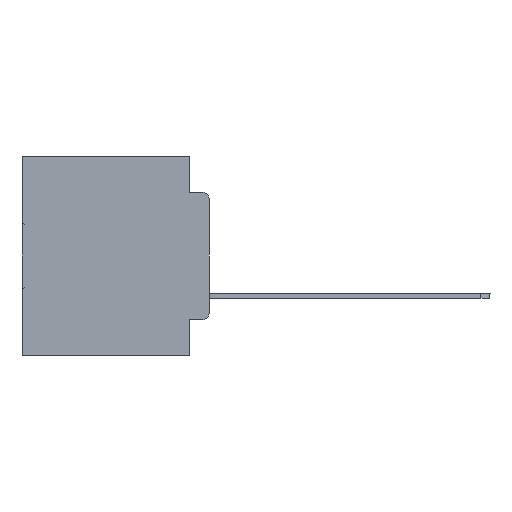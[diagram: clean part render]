
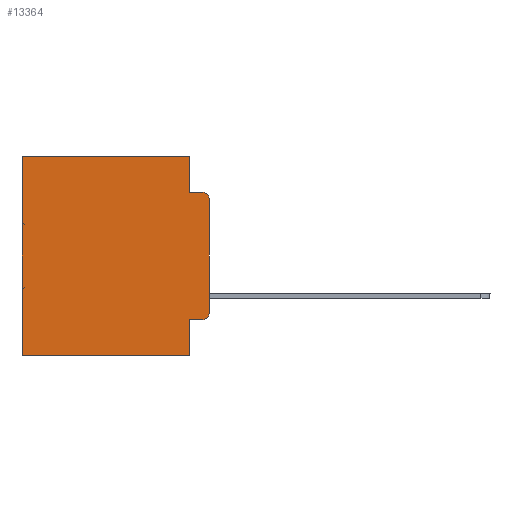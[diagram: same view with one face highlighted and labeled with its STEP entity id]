
A CAD part, left-side view. The second image highlights one B-rep face of the part: STEP entity #13364.
In plain terms, the highlighted planar face has unit normal (-1, 0, 0).
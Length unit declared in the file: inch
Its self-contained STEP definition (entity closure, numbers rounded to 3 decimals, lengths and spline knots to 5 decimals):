
#32 = LINE ( 'NONE', #24792, #26494 ) ;
#556 = ORIENTED_EDGE ( 'NONE', *, *, #33785, .F. ) ;
#729 = VECTOR ( 'NONE', #1368, 39.37008 ) ;
#1055 = DIRECTION ( 'NONE',  ( 0., 0., -1. ) ) ;
#1368 = DIRECTION ( 'NONE',  ( 0., 1., 0. ) ) ;
#2837 = LINE ( 'NONE', #18769, #14539 ) ;
#3476 = CARTESIAN_POINT ( 'NONE',  ( 0.298, 0.051, 0. ) ) ;
#3551 = CIRCLE ( 'NONE', #8074, 0.02 ) ;
#4330 = FACE_OUTER_BOUND ( 'NONE', #20759, .T. ) ;
#4646 = CARTESIAN_POINT ( 'NONE',  ( 0.298, 0.473, -0.5 ) ) ;
#4681 = AXIS2_PLACEMENT_3D ( 'NONE', #16268, #11324, #32523 ) ;
#4830 = DIRECTION ( 'NONE',  ( 1., 0., 0. ) ) ;
#4933 = CARTESIAN_POINT ( 'NONE',  ( 0.298, 0.02, -0.1085 ) ) ;
#5260 = ORIENTED_EDGE ( 'NONE', *, *, #27398, .F. ) ;
#5431 = LINE ( 'NONE', #3476, #23347 ) ;
#5491 = LINE ( 'NONE', #26901, #16795 ) ;
#6513 = VERTEX_POINT ( 'NONE', #16543 ) ;
#7020 = VERTEX_POINT ( 'NONE', #18983 ) ;
#8074 = AXIS2_PLACEMENT_3D ( 'NONE', #4933, #21043, #26337 ) ;
#9026 = CARTESIAN_POINT ( 'NONE',  ( 0.298, 0.473, 0. ) ) ;
#9737 = DIRECTION ( 'NONE',  ( 0., -1., 0. ) ) ;
#10448 = ORIENTED_EDGE ( 'NONE', *, *, #18953, .T. ) ;
#10665 = ORIENTED_EDGE ( 'NONE', *, *, #31456, .T. ) ;
#11016 = DIRECTION ( 'NONE',  ( 0., 1., 0. ) ) ;
#11118 = DIRECTION ( 'NONE',  ( 0., 0., -1. ) ) ;
#11324 = DIRECTION ( 'NONE',  ( -1., 0., 0. ) ) ;
#11407 = EDGE_CURVE ( 'NONE', #6513, #18928, #27294, .T. ) ;
#11514 = EDGE_CURVE ( 'NONE', #29895, #21654, #14820, .T. ) ;
#11563 = DIRECTION ( 'NONE',  ( 0., -1., 0. ) ) ;
#13364 = ADVANCED_FACE ( 'NONE', ( #4330 ), #15144, .F. ) ;
#13411 = VERTEX_POINT ( 'NONE', #17763 ) ;
#13927 = VERTEX_POINT ( 'NONE', #27042 ) ;
#14539 = VECTOR ( 'NONE', #20902, 39.37008 ) ;
#14692 = VECTOR ( 'NONE', #11563, 39.37008 ) ;
#14820 = LINE ( 'NONE', #25604, #729 ) ;
#15144 = PLANE ( 'NONE',  #18260 ) ;
#15481 = VERTEX_POINT ( 'NONE', #19646 ) ;
#15750 = LINE ( 'NONE', #31656, #22072 ) ;
#16268 = CARTESIAN_POINT ( 'NONE',  ( 0.298, 0.02, -0.3915 ) ) ;
#16543 = CARTESIAN_POINT ( 'NONE',  ( 0.298, 0.02, -0.4115 ) ) ;
#16795 = VECTOR ( 'NONE', #18418, 39.37008 ) ;
#17095 = ORIENTED_EDGE ( 'NONE', *, *, #33346, .T. ) ;
#17763 = CARTESIAN_POINT ( 'NONE',  ( 0.298, 0.02, -0.0885 ) ) ;
#18260 = AXIS2_PLACEMENT_3D ( 'NONE', #25920, #4830, #23417 ) ;
#18418 = DIRECTION ( 'NONE',  ( 0., 0., -1. ) ) ;
#18718 = ORIENTED_EDGE ( 'NONE', *, *, #11407, .T. ) ;
#18769 = CARTESIAN_POINT ( 'NONE',  ( 0.298, 0., 0. ) ) ;
#18787 = ORIENTED_EDGE ( 'NONE', *, *, #27328, .F. ) ;
#18928 = VERTEX_POINT ( 'NONE', #24437 ) ;
#18953 = EDGE_CURVE ( 'NONE', #26136, #27633, #32, .T. ) ;
#18983 = CARTESIAN_POINT ( 'NONE',  ( 0.298, 0.051, -0.0885 ) ) ;
#19646 = CARTESIAN_POINT ( 'NONE',  ( 0.298, 0.051, -0.4115 ) ) ;
#19843 = LINE ( 'NONE', #27649, #14692 ) ;
#20539 = EDGE_CURVE ( 'NONE', #7020, #13411, #15750, .T. ) ;
#20759 = EDGE_LOOP ( 'NONE', ( #5260, #17095, #34545, #556, #10448, #20967, #25933, #18787, #10665, #18718 ) ) ;
#20902 = DIRECTION ( 'NONE',  ( 0., 0., -1. ) ) ;
#20967 = ORIENTED_EDGE ( 'NONE', *, *, #31935, .T. ) ;
#21043 = DIRECTION ( 'NONE',  ( -1., 0., 0. ) ) ;
#21654 = VERTEX_POINT ( 'NONE', #4646 ) ;
#22072 = VECTOR ( 'NONE', #9737, 39.37008 ) ;
#23347 = VECTOR ( 'NONE', #11118, 39.37008 ) ;
#23417 = DIRECTION ( 'NONE',  ( 0., 0., -1. ) ) ;
#24437 = CARTESIAN_POINT ( 'NONE',  ( 0.298, 0., -0.3915 ) ) ;
#24792 = CARTESIAN_POINT ( 'NONE',  ( 0.298, 0., 0. ) ) ;
#24872 = VECTOR ( 'NONE', #1055, 39.37008 ) ;
#25461 = LINE ( 'NONE', #9026, #24872 ) ;
#25604 = CARTESIAN_POINT ( 'NONE',  ( 0.298, 0., -0.5 ) ) ;
#25625 = CARTESIAN_POINT ( 'NONE',  ( 0.298, 0.473, 0. ) ) ;
#25889 = CARTESIAN_POINT ( 'NONE',  ( 0.298, 0.051, -0.5 ) ) ;
#25920 = CARTESIAN_POINT ( 'NONE',  ( 0.298, 0., 0. ) ) ;
#25933 = ORIENTED_EDGE ( 'NONE', *, *, #11514, .F. ) ;
#26136 = VERTEX_POINT ( 'NONE', #33087 ) ;
#26337 = DIRECTION ( 'NONE',  ( 0., 0., -1. ) ) ;
#26494 = VECTOR ( 'NONE', #11016, 39.37008 ) ;
#26901 = CARTESIAN_POINT ( 'NONE',  ( 0.298, 0.051, 0. ) ) ;
#27042 = CARTESIAN_POINT ( 'NONE',  ( 0.298, 0., -0.1085 ) ) ;
#27294 = CIRCLE ( 'NONE', #4681, 0.02 ) ;
#27328 = EDGE_CURVE ( 'NONE', #15481, #29895, #5491, .T. ) ;
#27398 = EDGE_CURVE ( 'NONE', #13927, #18928, #2837, .T. ) ;
#27633 = VERTEX_POINT ( 'NONE', #25625 ) ;
#27649 = CARTESIAN_POINT ( 'NONE',  ( 0.298, 0.051, -0.4115 ) ) ;
#29895 = VERTEX_POINT ( 'NONE', #25889 ) ;
#31456 = EDGE_CURVE ( 'NONE', #15481, #6513, #19843, .T. ) ;
#31656 = CARTESIAN_POINT ( 'NONE',  ( 0.298, 0.051, -0.0885 ) ) ;
#31935 = EDGE_CURVE ( 'NONE', #27633, #21654, #25461, .T. ) ;
#32523 = DIRECTION ( 'NONE',  ( 0., 0., -1. ) ) ;
#33087 = CARTESIAN_POINT ( 'NONE',  ( 0.298, 0.051, 0. ) ) ;
#33346 = EDGE_CURVE ( 'NONE', #13927, #13411, #3551, .T. ) ;
#33785 = EDGE_CURVE ( 'NONE', #26136, #7020, #5431, .T. ) ;
#34545 = ORIENTED_EDGE ( 'NONE', *, *, #20539, .F. ) ;
